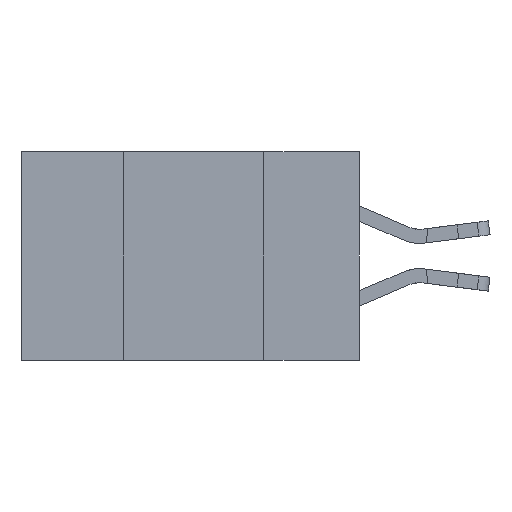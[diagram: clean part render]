
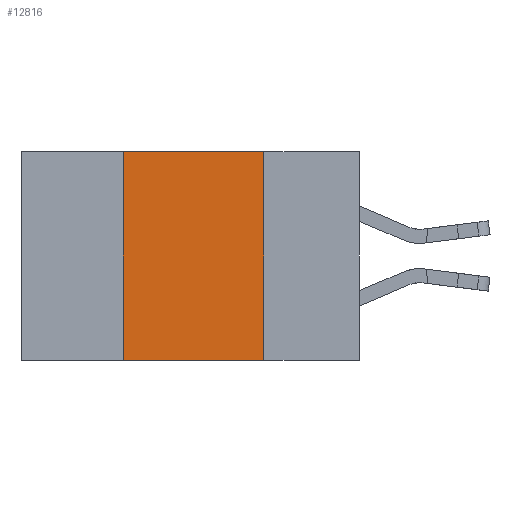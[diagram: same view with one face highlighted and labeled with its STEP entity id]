
A CAD part, left-side view. The second image highlights one B-rep face of the part: STEP entity #12816.
In plain terms, the highlighted planar face has unit normal (-1, 0, 0).
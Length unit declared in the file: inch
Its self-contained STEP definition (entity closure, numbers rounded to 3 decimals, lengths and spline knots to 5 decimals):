
#95 = LINE ( 'NONE', #7113, #16306 ) ;
#392 = AXIS2_PLACEMENT_3D ( 'NONE', #2055, #14458, #12852 ) ;
#572 = LINE ( 'NONE', #8503, #10270 ) ;
#1954 = CARTESIAN_POINT ( 'NONE',  ( 0., 0.17, -0.37 ) ) ;
#2055 = CARTESIAN_POINT ( 'NONE',  ( 0., 0.6, 0. ) ) ;
#2325 = EDGE_CURVE ( 'NONE', #14508, #2650, #572, .T. ) ;
#2650 = VERTEX_POINT ( 'NONE', #9568 ) ;
#2831 = ORIENTED_EDGE ( 'NONE', *, *, #12609, .F. ) ;
#3063 = ORIENTED_EDGE ( 'NONE', *, *, #2325, .F. ) ;
#3334 = ORIENTED_EDGE ( 'NONE', *, *, #8734, .T. ) ;
#4116 = ORIENTED_EDGE ( 'NONE', *, *, #12833, .F. ) ;
#6001 = DIRECTION ( 'NONE',  ( 0., 0., 1. ) ) ;
#6059 = CARTESIAN_POINT ( 'NONE',  ( 0., 0.17, 0. ) ) ;
#6322 = CARTESIAN_POINT ( 'NONE',  ( 0., 0.17, 0. ) ) ;
#7113 = CARTESIAN_POINT ( 'NONE',  ( 0., 0.6, 0. ) ) ;
#7329 = CARTESIAN_POINT ( 'NONE',  ( 0., 0.6, -0.37 ) ) ;
#8503 = CARTESIAN_POINT ( 'NONE',  ( 0., 0.42, 0. ) ) ;
#8734 = EDGE_CURVE ( 'NONE', #14508, #17602, #12513, .T. ) ;
#9014 = FACE_OUTER_BOUND ( 'NONE', #14741, .T. ) ;
#9568 = CARTESIAN_POINT ( 'NONE',  ( 0., 0.42, 0. ) ) ;
#10088 = PLANE ( 'NONE',  #392 ) ;
#10270 = VECTOR ( 'NONE', #6001, 39.37008 ) ;
#10380 = VECTOR ( 'NONE', #11509, 39.37008 ) ;
#11424 = VECTOR ( 'NONE', #14136, 39.37008 ) ;
#11509 = DIRECTION ( 'NONE',  ( 0., 0., -1. ) ) ;
#12513 = LINE ( 'NONE', #7329, #11424 ) ;
#12609 = EDGE_CURVE ( 'NONE', #2650, #14180, #95, .T. ) ;
#12682 = DIRECTION ( 'NONE',  ( 0., -1., 0. ) ) ;
#12816 = ADVANCED_FACE ( 'NONE', ( #9014 ), #10088, .F. ) ;
#12833 = EDGE_CURVE ( 'NONE', #14180, #17602, #13121, .T. ) ;
#12852 = DIRECTION ( 'NONE',  ( 0., 0., -1. ) ) ;
#13121 = LINE ( 'NONE', #6059, #10380 ) ;
#14136 = DIRECTION ( 'NONE',  ( 0., -1., 0. ) ) ;
#14180 = VERTEX_POINT ( 'NONE', #6322 ) ;
#14458 = DIRECTION ( 'NONE',  ( 1., 0., 0. ) ) ;
#14508 = VERTEX_POINT ( 'NONE', #16913 ) ;
#14741 = EDGE_LOOP ( 'NONE', ( #4116, #2831, #3063, #3334 ) ) ;
#16306 = VECTOR ( 'NONE', #12682, 39.37008 ) ;
#16913 = CARTESIAN_POINT ( 'NONE',  ( 0., 0.42, -0.37 ) ) ;
#17602 = VERTEX_POINT ( 'NONE', #1954 ) ;
